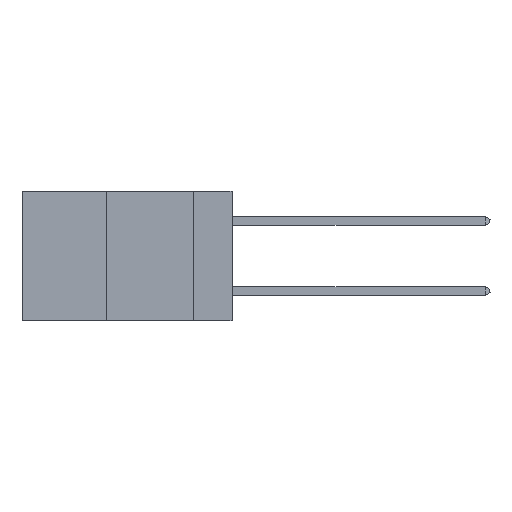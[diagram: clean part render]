
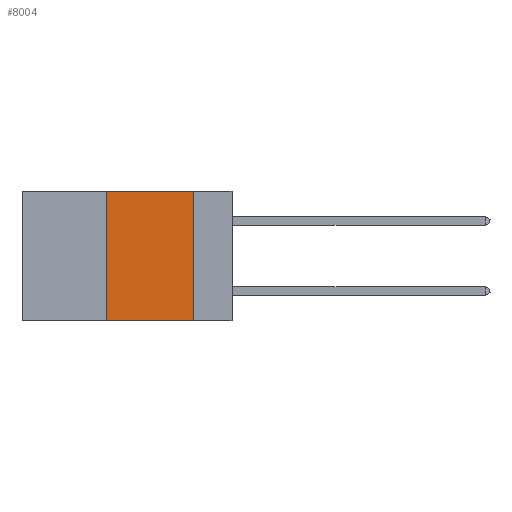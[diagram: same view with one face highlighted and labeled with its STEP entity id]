
A CAD part, left-side view. The second image highlights one B-rep face of the part: STEP entity #8004.
In plain terms, the highlighted planar face has unit normal (-1, 0, 0).
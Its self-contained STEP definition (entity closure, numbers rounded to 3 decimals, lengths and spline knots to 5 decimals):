
#1021 = ORIENTED_EDGE ( 'NONE', *, *, #37948, .F. ) ;
#1282 = EDGE_CURVE ( 'NONE', #6793, #18287, #42405, .T. ) ;
#3479 = VECTOR ( 'NONE', #14842, 39.37008 ) ;
#5366 = VECTOR ( 'NONE', #13378, 39.37008 ) ;
#6793 = VERTEX_POINT ( 'NONE', #9761 ) ;
#7510 = ORIENTED_EDGE ( 'NONE', *, *, #36914, .F. ) ;
#8004 = ADVANCED_FACE ( 'NONE', ( #14302 ), #19027, .F. ) ;
#9374 = VERTEX_POINT ( 'NONE', #23127 ) ;
#9761 = CARTESIAN_POINT ( 'NONE',  ( 0., 0.36, -0.37 ) ) ;
#12944 = VECTOR ( 'NONE', #34315, 39.37008 ) ;
#13378 = DIRECTION ( 'NONE',  ( 0., -1., 0. ) ) ;
#14302 = FACE_OUTER_BOUND ( 'NONE', #15414, .T. ) ;
#14842 = DIRECTION ( 'NONE',  ( 0., 0., -1. ) ) ;
#15414 = EDGE_LOOP ( 'NONE', ( #7510, #1021, #37919, #36813 ) ) ;
#16183 = DIRECTION ( 'NONE',  ( 0., 0., -1. ) ) ;
#16500 = EDGE_CURVE ( 'NONE', #6793, #9374, #41766, .T. ) ;
#18287 = VERTEX_POINT ( 'NONE', #33101 ) ;
#19027 = PLANE ( 'NONE',  #24780 ) ;
#19764 = LINE ( 'NONE', #29095, #3479 ) ;
#23127 = CARTESIAN_POINT ( 'NONE',  ( 0., 0.36, 0. ) ) ;
#24780 = AXIS2_PLACEMENT_3D ( 'NONE', #33566, #33706, #16183 ) ;
#27613 = CARTESIAN_POINT ( 'NONE',  ( 0., 0.6, -0.37 ) ) ;
#29095 = CARTESIAN_POINT ( 'NONE',  ( 0., 0.11, 0. ) ) ;
#30729 = CARTESIAN_POINT ( 'NONE',  ( 0., 0.6, 0. ) ) ;
#33101 = CARTESIAN_POINT ( 'NONE',  ( 0., 0.11, -0.37 ) ) ;
#33516 = CARTESIAN_POINT ( 'NONE',  ( 0., 0.36, 0. ) ) ;
#33566 = CARTESIAN_POINT ( 'NONE',  ( 0., 0.6, 0. ) ) ;
#33706 = DIRECTION ( 'NONE',  ( 1., 0., 0. ) ) ;
#34315 = DIRECTION ( 'NONE',  ( 0., -1., 0. ) ) ;
#34982 = VERTEX_POINT ( 'NONE', #43780 ) ;
#36813 = ORIENTED_EDGE ( 'NONE', *, *, #1282, .T. ) ;
#36914 = EDGE_CURVE ( 'NONE', #34982, #18287, #19764, .T. ) ;
#37838 = VECTOR ( 'NONE', #40761, 39.37008 ) ;
#37919 = ORIENTED_EDGE ( 'NONE', *, *, #16500, .F. ) ;
#37948 = EDGE_CURVE ( 'NONE', #9374, #34982, #43822, .T. ) ;
#40761 = DIRECTION ( 'NONE',  ( 0., 0., 1. ) ) ;
#41766 = LINE ( 'NONE', #33516, #37838 ) ;
#42405 = LINE ( 'NONE', #27613, #5366 ) ;
#43780 = CARTESIAN_POINT ( 'NONE',  ( 0., 0.11, 0. ) ) ;
#43822 = LINE ( 'NONE', #30729, #12944 ) ;
